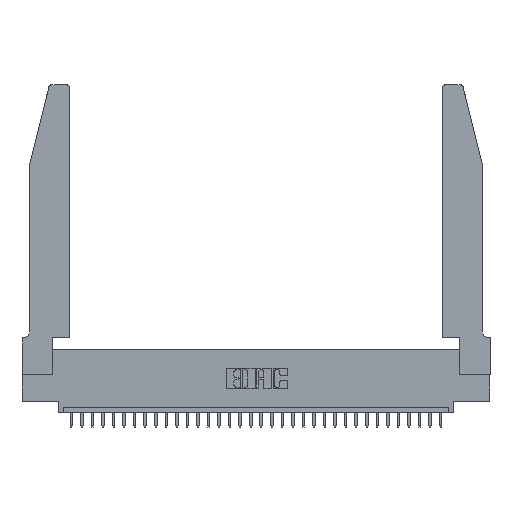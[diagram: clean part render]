
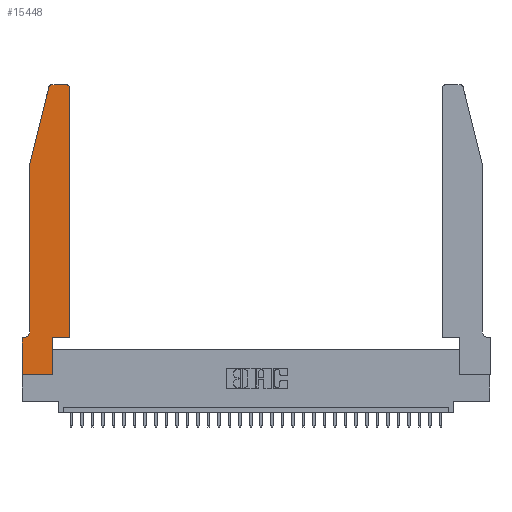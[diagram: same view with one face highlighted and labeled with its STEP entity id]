
A CAD part, top view. The second image highlights one B-rep face of the part: STEP entity #15448.
In plain terms, the highlighted planar face has unit normal (0, 0, 1).
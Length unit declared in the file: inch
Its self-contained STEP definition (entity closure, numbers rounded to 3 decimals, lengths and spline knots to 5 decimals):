
#20 = LINE ( 'NONE', #13569, #5969 ) ;
#726 = DIRECTION ( 'NONE',  ( -1., 0., 0. ) ) ;
#1255 = VERTEX_POINT ( 'NONE', #28674 ) ;
#1404 = ORIENTED_EDGE ( 'NONE', *, *, #11391, .T. ) ;
#1432 = LINE ( 'NONE', #26478, #3798 ) ;
#1510 = VERTEX_POINT ( 'NONE', #1664 ) ;
#1626 = EDGE_CURVE ( 'NONE', #17158, #14900, #1432, .T. ) ;
#1664 = CARTESIAN_POINT ( 'NONE',  ( 0.284, 2.75, 0.37 ) ) ;
#2237 = VECTOR ( 'NONE', #8092, 39.37008 ) ;
#2279 = EDGE_CURVE ( 'NONE', #10577, #14868, #22028, .T. ) ;
#3741 = DIRECTION ( 'NONE',  ( 1., 0., 0. ) ) ;
#3798 = VECTOR ( 'NONE', #14040, 39.37008 ) ;
#3905 = EDGE_CURVE ( 'NONE', #24831, #1255, #12506, .T. ) ;
#5682 = EDGE_CURVE ( 'NONE', #29112, #24831, #12630, .T. ) ;
#5796 = AXIS2_PLACEMENT_3D ( 'NONE', #32583, #11389, #16712 ) ;
#5969 = VECTOR ( 'NONE', #28419, 39.37008 ) ;
#6135 = ORIENTED_EDGE ( 'NONE', *, *, #22430, .T. ) ;
#6463 = FACE_OUTER_BOUND ( 'NONE', #15801, .T. ) ;
#6763 = VECTOR ( 'NONE', #24256, 39.37008 ) ;
#7004 = VECTOR ( 'NONE', #19248, 39.37008 ) ;
#7064 = CARTESIAN_POINT ( 'NONE',  ( 0.25487, 2.72718, 0.37 ) ) ;
#7817 = ORIENTED_EDGE ( 'NONE', *, *, #2279, .T. ) ;
#8092 = DIRECTION ( 'NONE',  ( 0., -1., 0. ) ) ;
#8538 = CARTESIAN_POINT ( 'NONE',  ( 0.0755, 2., 0.37 ) ) ;
#8543 = CARTESIAN_POINT ( 'NONE',  ( 0., 0., 0.37 ) ) ;
#8711 = AXIS2_PLACEMENT_3D ( 'NONE', #13015, #20548, #726 ) ;
#8775 = DIRECTION ( 'NONE',  ( 0., 0., 1. ) ) ;
#9312 = ORIENTED_EDGE ( 'NONE', *, *, #1626, .T. ) ;
#9481 = VECTOR ( 'NONE', #28399, 39.37008 ) ;
#9890 = CARTESIAN_POINT ( 'NONE',  ( 0.4505, 0.35, 0.37 ) ) ;
#10577 = VERTEX_POINT ( 'NONE', #22783 ) ;
#11389 = DIRECTION ( 'NONE',  ( 0., 0., 1. ) ) ;
#11391 = EDGE_CURVE ( 'NONE', #14868, #22223, #18164, .T. ) ;
#11621 = ORIENTED_EDGE ( 'NONE', *, *, #23067, .T. ) ;
#12262 = EDGE_CURVE ( 'NONE', #27136, #10577, #29914, .T. ) ;
#12494 = VERTEX_POINT ( 'NONE', #12570 ) ;
#12506 = LINE ( 'NONE', #8538, #6763 ) ;
#12570 = CARTESIAN_POINT ( 'NONE',  ( 0., 0., 0.37 ) ) ;
#12630 = LINE ( 'NONE', #23141, #29178 ) ;
#13015 = CARTESIAN_POINT ( 'NONE',  ( 0.0055, 0.42, 0.37 ) ) ;
#13260 = EDGE_CURVE ( 'NONE', #1255, #17158, #15264, .T. ) ;
#13569 = CARTESIAN_POINT ( 'NONE',  ( 0., 0., 0.37 ) ) ;
#14020 = VECTOR ( 'NONE', #22244, 39.37008 ) ;
#14040 = DIRECTION ( 'NONE',  ( -1., 0., 0. ) ) ;
#14075 = CARTESIAN_POINT ( 'NONE',  ( 0.2865, 0.35, 0.37 ) ) ;
#14140 = CARTESIAN_POINT ( 'NONE',  ( 0.4205, 2.75, 0.37 ) ) ;
#14868 = VERTEX_POINT ( 'NONE', #26098 ) ;
#14900 = VERTEX_POINT ( 'NONE', #22350 ) ;
#15264 = CIRCLE ( 'NONE', #8711, 0.07 ) ;
#15448 = ADVANCED_FACE ( 'NONE', ( #6463 ), #24982, .T. ) ;
#15772 = DIRECTION ( 'NONE',  ( -0.239, -0.971, 0. ) ) ;
#15801 = EDGE_LOOP ( 'NONE', ( #17835, #6135, #23864, #24064, #23553, #9312, #11621, #22316, #31363, #7817, #1404, #23485 ) ) ;
#16455 = CARTESIAN_POINT ( 'NONE',  ( 0.284, 2.72, 0.37 ) ) ;
#16712 = DIRECTION ( 'NONE',  ( 1., 0., 0. ) ) ;
#17082 = AXIS2_PLACEMENT_3D ( 'NONE', #16455, #8775, #3741 ) ;
#17117 = EDGE_CURVE ( 'NONE', #12494, #27136, #20, .T. ) ;
#17158 = VERTEX_POINT ( 'NONE', #20919 ) ;
#17835 = ORIENTED_EDGE ( 'NONE', *, *, #30757, .T. ) ;
#17995 = CIRCLE ( 'NONE', #18165, 0.03 ) ;
#18164 = LINE ( 'NONE', #9890, #9481 ) ;
#18165 = AXIS2_PLACEMENT_3D ( 'NONE', #27508, #32276, #30032 ) ;
#18503 = VECTOR ( 'NONE', #24896, 39.37008 ) ;
#19248 = DIRECTION ( 'NONE',  ( 0., 1., 0. ) ) ;
#20163 = CARTESIAN_POINT ( 'NONE',  ( 0.4505, 2.72, 0.37 ) ) ;
#20482 = LINE ( 'NONE', #8543, #2237 ) ;
#20548 = DIRECTION ( 'NONE',  ( 0., 0., -1. ) ) ;
#20655 = LINE ( 'NONE', #27015, #14020 ) ;
#20919 = CARTESIAN_POINT ( 'NONE',  ( 0.0055, 0.35, 0.37 ) ) ;
#22028 = LINE ( 'NONE', #22343, #18503 ) ;
#22223 = VERTEX_POINT ( 'NONE', #20163 ) ;
#22244 = DIRECTION ( 'NONE',  ( -1., 0., 0. ) ) ;
#22316 = ORIENTED_EDGE ( 'NONE', *, *, #17117, .T. ) ;
#22343 = CARTESIAN_POINT ( 'NONE',  ( 0.4505, 0.35, 0.37 ) ) ;
#22350 = CARTESIAN_POINT ( 'NONE',  ( 0., 0.35, 0.37 ) ) ;
#22430 = EDGE_CURVE ( 'NONE', #1510, #29112, #28038, .T. ) ;
#22783 = CARTESIAN_POINT ( 'NONE',  ( 0.2865, 0.35, 0.37 ) ) ;
#23067 = EDGE_CURVE ( 'NONE', #14900, #12494, #20482, .T. ) ;
#23141 = CARTESIAN_POINT ( 'NONE',  ( 0.0755, 2., 0.37 ) ) ;
#23485 = ORIENTED_EDGE ( 'NONE', *, *, #25581, .T. ) ;
#23553 = ORIENTED_EDGE ( 'NONE', *, *, #13260, .T. ) ;
#23864 = ORIENTED_EDGE ( 'NONE', *, *, #5682, .T. ) ;
#24064 = ORIENTED_EDGE ( 'NONE', *, *, #3905, .T. ) ;
#24256 = DIRECTION ( 'NONE',  ( 0., -1., 0. ) ) ;
#24831 = VERTEX_POINT ( 'NONE', #31885 ) ;
#24896 = DIRECTION ( 'NONE',  ( 1., 0., 0. ) ) ;
#24982 = PLANE ( 'NONE',  #5796 ) ;
#25581 = EDGE_CURVE ( 'NONE', #22223, #26144, #17995, .T. ) ;
#26098 = CARTESIAN_POINT ( 'NONE',  ( 0.4505, 0.35, 0.37 ) ) ;
#26144 = VERTEX_POINT ( 'NONE', #14140 ) ;
#26478 = CARTESIAN_POINT ( 'NONE',  ( 0.0755, 0.35, 0.37 ) ) ;
#27015 = CARTESIAN_POINT ( 'NONE',  ( 0.2605, 2.75, 0.37 ) ) ;
#27136 = VERTEX_POINT ( 'NONE', #27606 ) ;
#27508 = CARTESIAN_POINT ( 'NONE',  ( 0.4205, 2.72, 0.37 ) ) ;
#27606 = CARTESIAN_POINT ( 'NONE',  ( 0.2865, 0., 0.37 ) ) ;
#28038 = CIRCLE ( 'NONE', #17082, 0.03 ) ;
#28399 = DIRECTION ( 'NONE',  ( 0., 1., 0. ) ) ;
#28419 = DIRECTION ( 'NONE',  ( 1., 0., 0. ) ) ;
#28674 = CARTESIAN_POINT ( 'NONE',  ( 0.0755, 0.42, 0.37 ) ) ;
#29112 = VERTEX_POINT ( 'NONE', #7064 ) ;
#29178 = VECTOR ( 'NONE', #15772, 39.37008 ) ;
#29914 = LINE ( 'NONE', #14075, #7004 ) ;
#30032 = DIRECTION ( 'NONE',  ( 1., 0., 0. ) ) ;
#30757 = EDGE_CURVE ( 'NONE', #26144, #1510, #20655, .T. ) ;
#31363 = ORIENTED_EDGE ( 'NONE', *, *, #12262, .T. ) ;
#31885 = CARTESIAN_POINT ( 'NONE',  ( 0.0755, 2., 0.37 ) ) ;
#32276 = DIRECTION ( 'NONE',  ( 0., 0., 1. ) ) ;
#32583 = CARTESIAN_POINT ( 'NONE',  ( 0., 0.35, 0.37 ) ) ;
